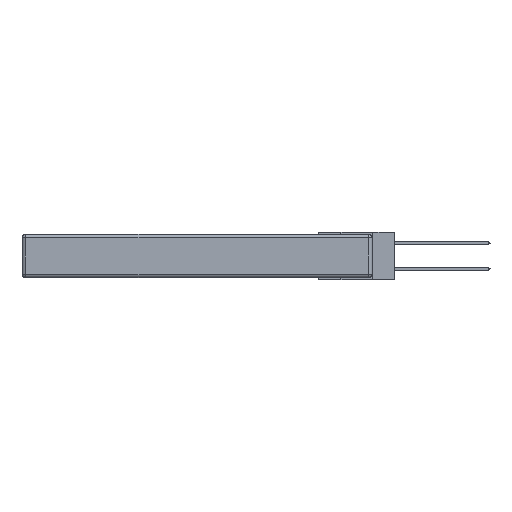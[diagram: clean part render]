
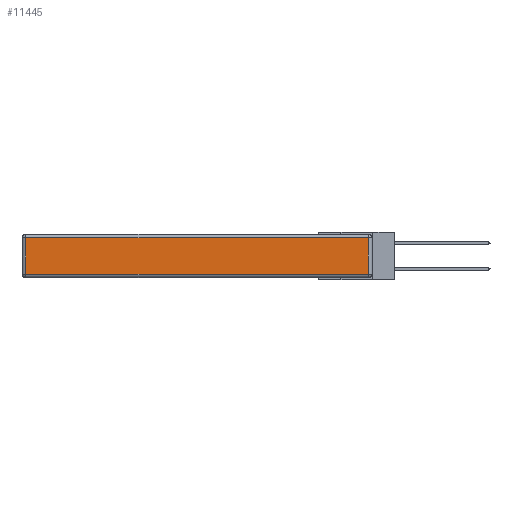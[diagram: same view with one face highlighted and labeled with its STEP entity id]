
A CAD part, left-side view. The second image highlights one B-rep face of the part: STEP entity #11445.
In plain terms, the highlighted planar face has unit normal (-1, 0, 0).
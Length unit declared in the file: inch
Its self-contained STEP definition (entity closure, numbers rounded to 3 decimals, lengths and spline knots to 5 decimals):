
#459 = FACE_OUTER_BOUND ( 'NONE', #5041, .T. ) ;
#853 = CARTESIAN_POINT ( 'NONE',  ( 0., 2.72, -0.313 ) ) ;
#920 = CARTESIAN_POINT ( 'NONE',  ( 0., 0.03, -0.343 ) ) ;
#1954 = CARTESIAN_POINT ( 'NONE',  ( 0., 0., -0.313 ) ) ;
#2276 = DIRECTION ( 'NONE',  ( 0., -1., 0. ) ) ;
#2465 = VECTOR ( 'NONE', #18894, 39.37008 ) ;
#3279 = ORIENTED_EDGE ( 'NONE', *, *, #25169, .T. ) ;
#3763 = AXIS2_PLACEMENT_3D ( 'NONE', #14149, #26866, #11232 ) ;
#5041 = EDGE_LOOP ( 'NONE', ( #8567, #28452, #3279, #25638 ) ) ;
#5994 = DIRECTION ( 'NONE',  ( 0., 0., 1. ) ) ;
#6045 = CARTESIAN_POINT ( 'NONE',  ( 0., 2.72, -0.343 ) ) ;
#6278 = CARTESIAN_POINT ( 'NONE',  ( 0., 0.03, -0.313 ) ) ;
#8567 = ORIENTED_EDGE ( 'NONE', *, *, #31178, .T. ) ;
#8575 = CARTESIAN_POINT ( 'NONE',  ( 0., 2.72, -0.03 ) ) ;
#11068 = DIRECTION ( 'NONE',  ( 0., 0., -1. ) ) ;
#11232 = DIRECTION ( 'NONE',  ( 0., 0., 1. ) ) ;
#11234 = CARTESIAN_POINT ( 'NONE',  ( 0., 2.75, -0.03 ) ) ;
#11387 = LINE ( 'NONE', #6045, #26878 ) ;
#11445 = ADVANCED_FACE ( 'NONE', ( #459 ), #19004, .T. ) ;
#11900 = VERTEX_POINT ( 'NONE', #6278 ) ;
#12448 = LINE ( 'NONE', #1954, #13256 ) ;
#13256 = VECTOR ( 'NONE', #2276, 39.37008 ) ;
#14149 = CARTESIAN_POINT ( 'NONE',  ( 0., 0., -0.343 ) ) ;
#16050 = EDGE_CURVE ( 'NONE', #17937, #19236, #11387, .T. ) ;
#16752 = CARTESIAN_POINT ( 'NONE',  ( 0., 0.03, -0.03 ) ) ;
#16808 = VERTEX_POINT ( 'NONE', #16752 ) ;
#17937 = VERTEX_POINT ( 'NONE', #8575 ) ;
#18243 = VECTOR ( 'NONE', #5994, 39.37008 ) ;
#18894 = DIRECTION ( 'NONE',  ( 0., 1., 0. ) ) ;
#19004 = PLANE ( 'NONE',  #3763 ) ;
#19236 = VERTEX_POINT ( 'NONE', #853 ) ;
#24957 = LINE ( 'NONE', #920, #18243 ) ;
#25102 = EDGE_CURVE ( 'NONE', #11900, #16808, #24957, .T. ) ;
#25169 = EDGE_CURVE ( 'NONE', #16808, #17937, #30156, .T. ) ;
#25638 = ORIENTED_EDGE ( 'NONE', *, *, #16050, .T. ) ;
#26866 = DIRECTION ( 'NONE',  ( -1., 0., 0. ) ) ;
#26878 = VECTOR ( 'NONE', #11068, 39.37008 ) ;
#28452 = ORIENTED_EDGE ( 'NONE', *, *, #25102, .T. ) ;
#30156 = LINE ( 'NONE', #11234, #2465 ) ;
#31178 = EDGE_CURVE ( 'NONE', #19236, #11900, #12448, .T. ) ;
